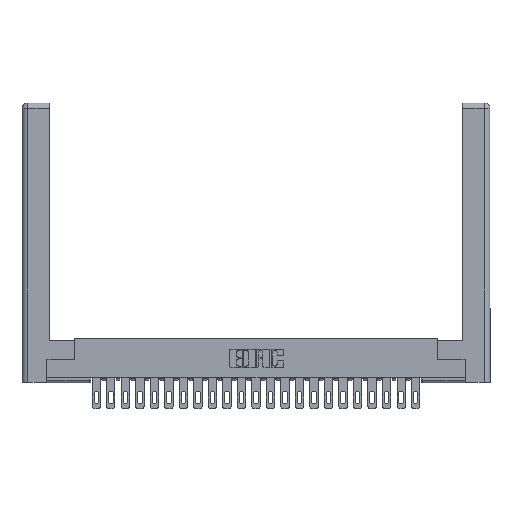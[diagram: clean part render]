
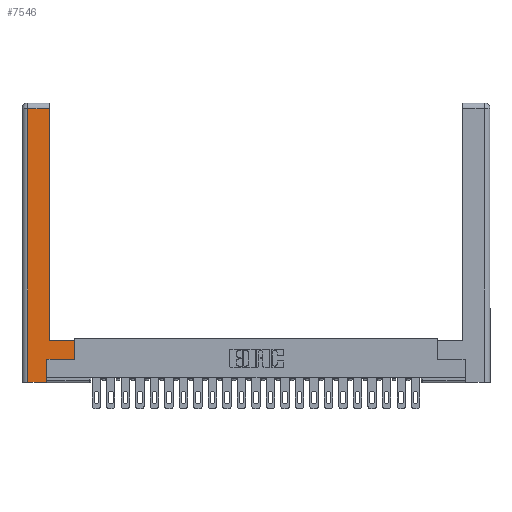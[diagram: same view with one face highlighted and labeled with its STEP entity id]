
A CAD part, top view. The second image highlights one B-rep face of the part: STEP entity #7546.
In plain terms, the highlighted planar face has unit normal (0, 0, 1).
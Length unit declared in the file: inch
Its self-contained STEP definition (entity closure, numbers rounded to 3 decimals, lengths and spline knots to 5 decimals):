
#491 = CARTESIAN_POINT ( 'NONE',  ( 0.295, 0.45, 0. ) ) ;
#513 = CARTESIAN_POINT ( 'NONE',  ( 0.565, 0.45, 0. ) ) ;
#803 = CARTESIAN_POINT ( 'NONE',  ( 0.565, 0.45, 0. ) ) ;
#1341 = LINE ( 'NONE', #18234, #15129 ) ;
#1728 = CARTESIAN_POINT ( 'NONE',  ( 0.295, 3., 0. ) ) ;
#1856 = VERTEX_POINT ( 'NONE', #19913 ) ;
#2870 = CARTESIAN_POINT ( 'NONE',  ( 0., 0., 0. ) ) ;
#3801 = ORIENTED_EDGE ( 'NONE', *, *, #13573, .T. ) ;
#4036 = VECTOR ( 'NONE', #23862, 39.37008 ) ;
#4565 = EDGE_LOOP ( 'NONE', ( #7069, #15382, #20868, #11772, #17773, #19549, #18988, #3801 ) ) ;
#4731 = DIRECTION ( 'NONE',  ( 0., 0., -1. ) ) ;
#5992 = LINE ( 'NONE', #13224, #13356 ) ;
#6340 = DIRECTION ( 'NONE',  ( 1., 0., 0. ) ) ;
#6447 = VERTEX_POINT ( 'NONE', #7044 ) ;
#7044 = CARTESIAN_POINT ( 'NONE',  ( 0.0615, 2.94, 0. ) ) ;
#7069 = ORIENTED_EDGE ( 'NONE', *, *, #17895, .T. ) ;
#7546 = ADVANCED_FACE ( 'NONE', ( #8992 ), #8689, .F. ) ;
#8689 = PLANE ( 'NONE',  #14643 ) ;
#8740 = EDGE_CURVE ( 'NONE', #8751, #6447, #20224, .T. ) ;
#8742 = LINE ( 'NONE', #21878, #11494 ) ;
#8751 = VERTEX_POINT ( 'NONE', #24281 ) ;
#8992 = FACE_OUTER_BOUND ( 'NONE', #4565, .T. ) ;
#9266 = LINE ( 'NONE', #17969, #4036 ) ;
#9561 = VECTOR ( 'NONE', #19376, 39.37008 ) ;
#10263 = VECTOR ( 'NONE', #20134, 39.37008 ) ;
#10328 = VERTEX_POINT ( 'NONE', #14270 ) ;
#10555 = CARTESIAN_POINT ( 'NONE',  ( 0.0615, 2.94, 0. ) ) ;
#11083 = CARTESIAN_POINT ( 'NONE',  ( 0.295, 0.45, 0. ) ) ;
#11225 = EDGE_CURVE ( 'NONE', #6447, #19188, #5992, .T. ) ;
#11494 = VECTOR ( 'NONE', #6340, 39.37008 ) ;
#11518 = EDGE_CURVE ( 'NONE', #1856, #10328, #8742, .T. ) ;
#11660 = EDGE_CURVE ( 'NONE', #10328, #14233, #16724, .T. ) ;
#11772 = ORIENTED_EDGE ( 'NONE', *, *, #16897, .T. ) ;
#12285 = CARTESIAN_POINT ( 'NONE',  ( 0.0615, 0., 0. ) ) ;
#13009 = VERTEX_POINT ( 'NONE', #16731 ) ;
#13224 = CARTESIAN_POINT ( 'NONE',  ( 0.0615, 0., 0. ) ) ;
#13356 = VECTOR ( 'NONE', #21136, 39.37008 ) ;
#13573 = EDGE_CURVE ( 'NONE', #14233, #23382, #19718, .T. ) ;
#14233 = VERTEX_POINT ( 'NONE', #803 ) ;
#14270 = CARTESIAN_POINT ( 'NONE',  ( 0.565, 0.245, 0. ) ) ;
#14576 = DIRECTION ( 'NONE',  ( -1., 0., 0. ) ) ;
#14643 = AXIS2_PLACEMENT_3D ( 'NONE', #2870, #4731, #24040 ) ;
#15129 = VECTOR ( 'NONE', #18072, 39.37008 ) ;
#15382 = ORIENTED_EDGE ( 'NONE', *, *, #8740, .T. ) ;
#16437 = DIRECTION ( 'NONE',  ( -1., 0., 0. ) ) ;
#16724 = LINE ( 'NONE', #513, #10263 ) ;
#16731 = CARTESIAN_POINT ( 'NONE',  ( 0.265, 0., 0. ) ) ;
#16897 = EDGE_CURVE ( 'NONE', #19188, #13009, #1341, .T. ) ;
#17439 = EDGE_CURVE ( 'NONE', #13009, #1856, #9266, .T. ) ;
#17495 = VECTOR ( 'NONE', #14576, 39.37008 ) ;
#17533 = LINE ( 'NONE', #1728, #9561 ) ;
#17773 = ORIENTED_EDGE ( 'NONE', *, *, #17439, .T. ) ;
#17895 = EDGE_CURVE ( 'NONE', #23382, #8751, #17533, .T. ) ;
#17969 = CARTESIAN_POINT ( 'NONE',  ( 0.265, 0.245, 0. ) ) ;
#18072 = DIRECTION ( 'NONE',  ( 1., 0., 0. ) ) ;
#18234 = CARTESIAN_POINT ( 'NONE',  ( 0.265, 0., 0. ) ) ;
#18988 = ORIENTED_EDGE ( 'NONE', *, *, #11660, .T. ) ;
#19188 = VERTEX_POINT ( 'NONE', #12285 ) ;
#19376 = DIRECTION ( 'NONE',  ( 0., 1., 0. ) ) ;
#19549 = ORIENTED_EDGE ( 'NONE', *, *, #11518, .T. ) ;
#19718 = LINE ( 'NONE', #491, #23389 ) ;
#19913 = CARTESIAN_POINT ( 'NONE',  ( 0.265, 0.245, 0. ) ) ;
#20134 = DIRECTION ( 'NONE',  ( 0., 1., 0. ) ) ;
#20224 = LINE ( 'NONE', #10555, #17495 ) ;
#20868 = ORIENTED_EDGE ( 'NONE', *, *, #11225, .T. ) ;
#21136 = DIRECTION ( 'NONE',  ( 0., -1., 0. ) ) ;
#21878 = CARTESIAN_POINT ( 'NONE',  ( 0.565, 0.245, 0. ) ) ;
#23382 = VERTEX_POINT ( 'NONE', #11083 ) ;
#23389 = VECTOR ( 'NONE', #16437, 39.37008 ) ;
#23862 = DIRECTION ( 'NONE',  ( 0., 1., 0. ) ) ;
#24040 = DIRECTION ( 'NONE',  ( -1., 0., 0. ) ) ;
#24281 = CARTESIAN_POINT ( 'NONE',  ( 0.295, 2.94, 0. ) ) ;
